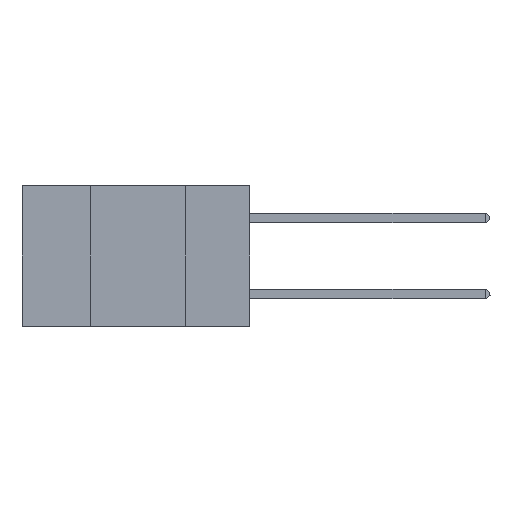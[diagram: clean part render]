
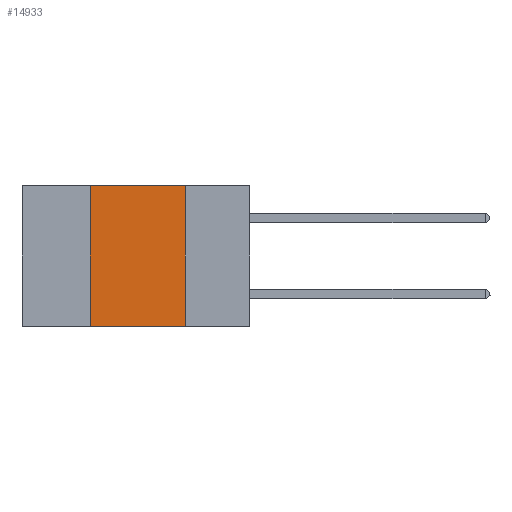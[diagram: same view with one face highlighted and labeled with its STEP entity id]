
A CAD part, left-side view. The second image highlights one B-rep face of the part: STEP entity #14933.
In plain terms, the highlighted planar face has unit normal (-1, 0, 0).
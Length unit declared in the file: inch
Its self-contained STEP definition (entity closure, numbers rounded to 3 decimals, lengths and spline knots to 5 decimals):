
#477 = VECTOR ( 'NONE', #3826, 39.37008 ) ;
#513 = CARTESIAN_POINT ( 'NONE',  ( 0., 0.17, 0. ) ) ;
#651 = CARTESIAN_POINT ( 'NONE',  ( 0., 0.6, 0. ) ) ;
#1233 = CARTESIAN_POINT ( 'NONE',  ( 0., 0.17, -0.37 ) ) ;
#2197 = LINE ( 'NONE', #14843, #17070 ) ;
#2616 = VERTEX_POINT ( 'NONE', #1233 ) ;
#2916 = AXIS2_PLACEMENT_3D ( 'NONE', #651, #8349, #8205 ) ;
#3005 = ORIENTED_EDGE ( 'NONE', *, *, #4352, .F. ) ;
#3723 = LINE ( 'NONE', #16801, #15640 ) ;
#3826 = DIRECTION ( 'NONE',  ( 0., 0., -1. ) ) ;
#4352 = EDGE_CURVE ( 'NONE', #12920, #14308, #3723, .T. ) ;
#4969 = VECTOR ( 'NONE', #10440, 39.37008 ) ;
#6083 = EDGE_CURVE ( 'NONE', #13189, #12920, #2197, .T. ) ;
#6297 = PLANE ( 'NONE',  #2916 ) ;
#6806 = ORIENTED_EDGE ( 'NONE', *, *, #15537, .F. ) ;
#6850 = CARTESIAN_POINT ( 'NONE',  ( 0., 0.6, -0.37 ) ) ;
#7813 = ORIENTED_EDGE ( 'NONE', *, *, #6083, .F. ) ;
#8205 = DIRECTION ( 'NONE',  ( 0., 0., -1. ) ) ;
#8349 = DIRECTION ( 'NONE',  ( 1., 0., 0. ) ) ;
#8775 = LINE ( 'NONE', #513, #477 ) ;
#9041 = CARTESIAN_POINT ( 'NONE',  ( 0., 0.42, -0.37 ) ) ;
#9637 = LINE ( 'NONE', #6850, #4969 ) ;
#10374 = DIRECTION ( 'NONE',  ( 0., -1., 0. ) ) ;
#10440 = DIRECTION ( 'NONE',  ( 0., -1., 0. ) ) ;
#10668 = EDGE_CURVE ( 'NONE', #13189, #2616, #9637, .T. ) ;
#12920 = VERTEX_POINT ( 'NONE', #17489 ) ;
#13121 = EDGE_LOOP ( 'NONE', ( #6806, #3005, #7813, #17686 ) ) ;
#13189 = VERTEX_POINT ( 'NONE', #9041 ) ;
#14308 = VERTEX_POINT ( 'NONE', #14997 ) ;
#14843 = CARTESIAN_POINT ( 'NONE',  ( 0., 0.42, 0. ) ) ;
#14933 = ADVANCED_FACE ( 'NONE', ( #18249 ), #6297, .F. ) ;
#14997 = CARTESIAN_POINT ( 'NONE',  ( 0., 0.17, 0. ) ) ;
#15537 = EDGE_CURVE ( 'NONE', #14308, #2616, #8775, .T. ) ;
#15640 = VECTOR ( 'NONE', #10374, 39.37008 ) ;
#16425 = DIRECTION ( 'NONE',  ( 0., 0., 1. ) ) ;
#16801 = CARTESIAN_POINT ( 'NONE',  ( 0., 0.6, 0. ) ) ;
#17070 = VECTOR ( 'NONE', #16425, 39.37008 ) ;
#17489 = CARTESIAN_POINT ( 'NONE',  ( 0., 0.42, 0. ) ) ;
#17686 = ORIENTED_EDGE ( 'NONE', *, *, #10668, .T. ) ;
#18249 = FACE_OUTER_BOUND ( 'NONE', #13121, .T. ) ;
